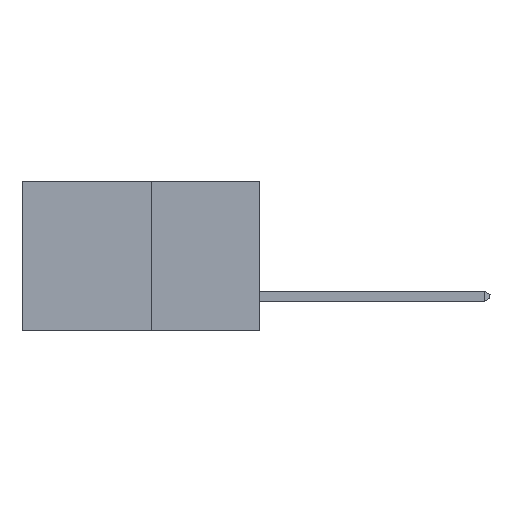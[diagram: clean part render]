
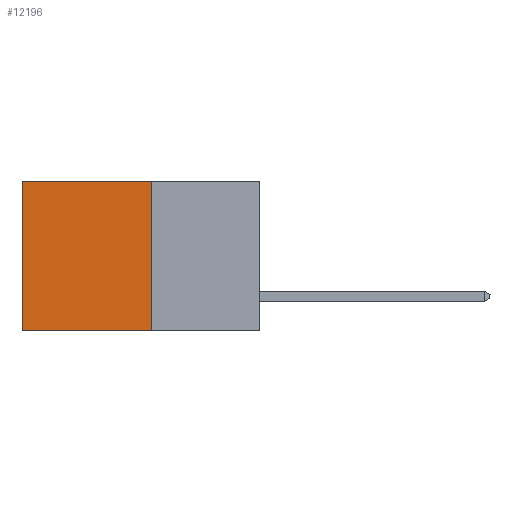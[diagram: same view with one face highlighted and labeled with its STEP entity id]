
A CAD part, left-side view. The second image highlights one B-rep face of the part: STEP entity #12196.
In plain terms, the highlighted planar face has unit normal (-1, 0, 0).
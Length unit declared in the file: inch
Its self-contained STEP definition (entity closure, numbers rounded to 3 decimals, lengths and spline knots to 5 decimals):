
#118 = AXIS2_PLACEMENT_3D ( 'NONE', #1714, #13943, #3516 ) ;
#198 = CARTESIAN_POINT ( 'NONE',  ( 0.277, 0.27, -0.37 ) ) ;
#1714 = CARTESIAN_POINT ( 'NONE',  ( 0.277, 0.27, -0.37 ) ) ;
#1984 = ORIENTED_EDGE ( 'NONE', *, *, #17331, .F. ) ;
#2113 = CARTESIAN_POINT ( 'NONE',  ( 0.277, 0.59, -0.37 ) ) ;
#2240 = EDGE_CURVE ( 'NONE', #20927, #8082, #5519, .T. ) ;
#2476 = EDGE_CURVE ( 'NONE', #21646, #10955, #18873, .T. ) ;
#3516 = DIRECTION ( 'NONE',  ( 0., 0., -1. ) ) ;
#3801 = CARTESIAN_POINT ( 'NONE',  ( 0.277, 0.27, -0.37 ) ) ;
#4167 = CARTESIAN_POINT ( 'NONE',  ( 0.277, 0.27, 0. ) ) ;
#4381 = VECTOR ( 'NONE', #5957, 39.37008 ) ;
#4393 = ORIENTED_EDGE ( 'NONE', *, *, #2240, .T. ) ;
#5052 = CARTESIAN_POINT ( 'NONE',  ( 0.277, 0.27, -0.37 ) ) ;
#5519 = LINE ( 'NONE', #9597, #6058 ) ;
#5666 = DIRECTION ( 'NONE',  ( 0., 0., -1. ) ) ;
#5957 = DIRECTION ( 'NONE',  ( 0., 1., 0. ) ) ;
#6058 = VECTOR ( 'NONE', #5666, 39.37008 ) ;
#6793 = DIRECTION ( 'NONE',  ( 0., 1., 0. ) ) ;
#8082 = VERTEX_POINT ( 'NONE', #2113 ) ;
#8930 = FACE_OUTER_BOUND ( 'NONE', #18325, .T. ) ;
#9046 = CARTESIAN_POINT ( 'NONE',  ( 0.277, 0.59, 0. ) ) ;
#9597 = CARTESIAN_POINT ( 'NONE',  ( 0.277, 0.59, -0.37 ) ) ;
#9864 = VECTOR ( 'NONE', #12247, 39.37008 ) ;
#10046 = EDGE_CURVE ( 'NONE', #21646, #20927, #18090, .T. ) ;
#10955 = VERTEX_POINT ( 'NONE', #3801 ) ;
#11327 = ORIENTED_EDGE ( 'NONE', *, *, #10046, .T. ) ;
#11577 = LINE ( 'NONE', #5052, #15582 ) ;
#12077 = CARTESIAN_POINT ( 'NONE',  ( 0.277, 0.27, 0. ) ) ;
#12196 = ADVANCED_FACE ( 'NONE', ( #8930 ), #12230, .F. ) ;
#12230 = PLANE ( 'NONE',  #118 ) ;
#12247 = DIRECTION ( 'NONE',  ( 0., 0., -1. ) ) ;
#13943 = DIRECTION ( 'NONE',  ( 1., 0., 0. ) ) ;
#15582 = VECTOR ( 'NONE', #6793, 39.37008 ) ;
#17331 = EDGE_CURVE ( 'NONE', #10955, #8082, #11577, .T. ) ;
#18090 = LINE ( 'NONE', #4167, #4381 ) ;
#18325 = EDGE_LOOP ( 'NONE', ( #4393, #1984, #20239, #11327 ) ) ;
#18873 = LINE ( 'NONE', #198, #9864 ) ;
#20239 = ORIENTED_EDGE ( 'NONE', *, *, #2476, .F. ) ;
#20927 = VERTEX_POINT ( 'NONE', #9046 ) ;
#21646 = VERTEX_POINT ( 'NONE', #12077 ) ;
